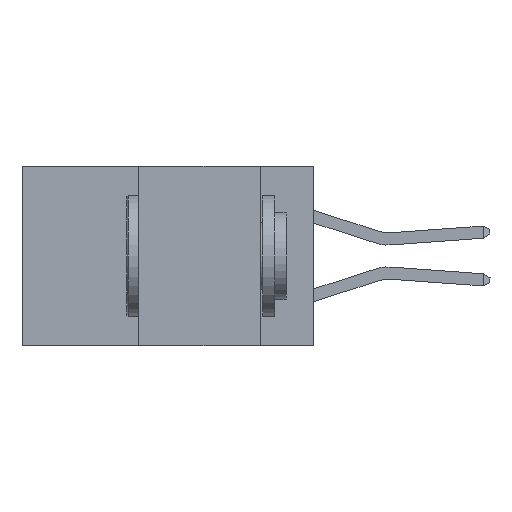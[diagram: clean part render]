
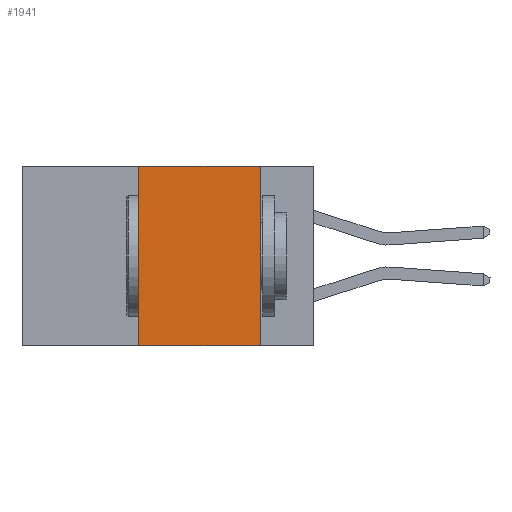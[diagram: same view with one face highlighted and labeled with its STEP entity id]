
A CAD part, left-side view. The second image highlights one B-rep face of the part: STEP entity #1941.
In plain terms, the highlighted planar face has unit normal (-1, 0, 0).
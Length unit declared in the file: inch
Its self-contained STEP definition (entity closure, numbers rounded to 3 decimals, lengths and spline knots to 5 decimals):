
#171 = DIRECTION ( 'NONE',  ( 0., 0., -1. ) ) ;
#193 = DIRECTION ( 'NONE',  ( 1., 0., 0. ) ) ;
#285 = CARTESIAN_POINT ( 'NONE',  ( 0., 0.6, 0. ) ) ;
#310 = PLANE ( 'NONE',  #5920 ) ;
#814 = VERTEX_POINT ( 'NONE', #19033 ) ;
#1341 = EDGE_LOOP ( 'NONE', ( #17174, #17387, #17701, #18632 ) ) ;
#1514 = VECTOR ( 'NONE', #21944, 39.37008 ) ;
#1586 = EDGE_CURVE ( 'NONE', #814, #16079, #17678, .T. ) ;
#1745 = DIRECTION ( 'NONE',  ( 0., -1., 0. ) ) ;
#1941 = ADVANCED_FACE ( 'NONE', ( #10267 ), #310, .F. ) ;
#4071 = VECTOR ( 'NONE', #6396, 39.37008 ) ;
#5920 = AXIS2_PLACEMENT_3D ( 'NONE', #285, #193, #171 ) ;
#6396 = DIRECTION ( 'NONE',  ( 0., 0., -1. ) ) ;
#6563 = CARTESIAN_POINT ( 'NONE',  ( 0., 0.11, 0. ) ) ;
#6627 = CARTESIAN_POINT ( 'NONE',  ( 0., 0.6, -0.37 ) ) ;
#8533 = VECTOR ( 'NONE', #20353, 39.37008 ) ;
#8575 = EDGE_CURVE ( 'NONE', #15472, #814, #19642, .T. ) ;
#9444 = VERTEX_POINT ( 'NONE', #19669 ) ;
#10267 = FACE_OUTER_BOUND ( 'NONE', #1341, .T. ) ;
#11781 = EDGE_CURVE ( 'NONE', #9444, #16079, #15678, .T. ) ;
#12005 = LINE ( 'NONE', #20365, #8533 ) ;
#13763 = CARTESIAN_POINT ( 'NONE',  ( 0., 0.11, -0.37 ) ) ;
#15472 = VERTEX_POINT ( 'NONE', #20260 ) ;
#15678 = LINE ( 'NONE', #6627, #1514 ) ;
#16079 = VERTEX_POINT ( 'NONE', #13763 ) ;
#17174 = ORIENTED_EDGE ( 'NONE', *, *, #1586, .F. ) ;
#17387 = ORIENTED_EDGE ( 'NONE', *, *, #8575, .F. ) ;
#17678 = LINE ( 'NONE', #6563, #4071 ) ;
#17701 = ORIENTED_EDGE ( 'NONE', *, *, #18477, .F. ) ;
#18477 = EDGE_CURVE ( 'NONE', #9444, #15472, #12005, .T. ) ;
#18632 = ORIENTED_EDGE ( 'NONE', *, *, #11781, .T. ) ;
#18732 = CARTESIAN_POINT ( 'NONE',  ( 0., 0.6, 0. ) ) ;
#19033 = CARTESIAN_POINT ( 'NONE',  ( 0., 0.11, 0. ) ) ;
#19111 = VECTOR ( 'NONE', #1745, 39.37008 ) ;
#19642 = LINE ( 'NONE', #18732, #19111 ) ;
#19669 = CARTESIAN_POINT ( 'NONE',  ( 0., 0.36, -0.37 ) ) ;
#20260 = CARTESIAN_POINT ( 'NONE',  ( 0., 0.36, 0. ) ) ;
#20353 = DIRECTION ( 'NONE',  ( 0., 0., 1. ) ) ;
#20365 = CARTESIAN_POINT ( 'NONE',  ( 0., 0.36, 0. ) ) ;
#21944 = DIRECTION ( 'NONE',  ( 0., -1., 0. ) ) ;
